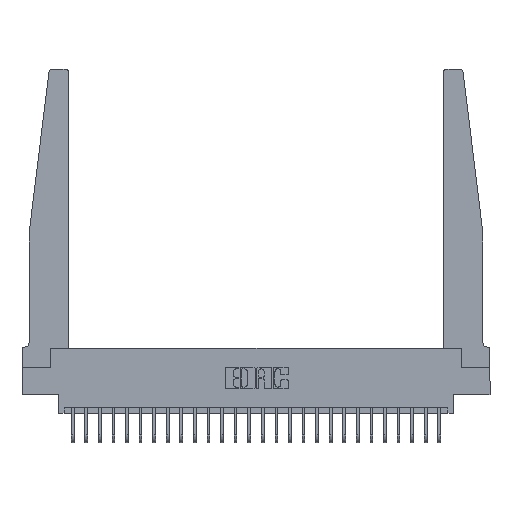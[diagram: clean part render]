
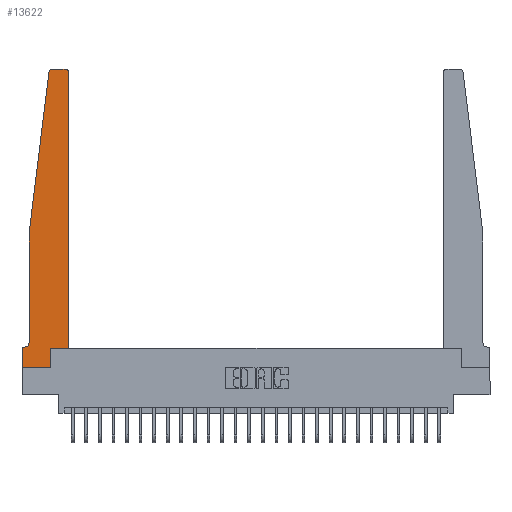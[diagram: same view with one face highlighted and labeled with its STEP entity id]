
A CAD part, top view. The second image highlights one B-rep face of the part: STEP entity #13622.
In plain terms, the highlighted planar face has unit normal (0, 0, 1).
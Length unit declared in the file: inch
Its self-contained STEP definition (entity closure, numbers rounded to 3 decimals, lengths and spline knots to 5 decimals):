
#13 = VERTEX_POINT ( 'NONE', #8820 ) ;
#181 = CIRCLE ( 'NONE', #4555, 0.03 ) ;
#565 = VERTEX_POINT ( 'NONE', #1072 ) ;
#1072 = CARTESIAN_POINT ( 'NONE',  ( 0.015, 0.1875, 0.37 ) ) ;
#1398 = DIRECTION ( 'NONE',  ( -1., 0., 0. ) ) ;
#1427 = EDGE_CURVE ( 'NONE', #3581, #565, #5714, .T. ) ;
#1668 = LINE ( 'NONE', #9292, #10512 ) ;
#1743 = VECTOR ( 'NONE', #21813, 39.37008 ) ;
#1884 = CARTESIAN_POINT ( 'NONE',  ( 0., 0.1875, 0.37 ) ) ;
#1920 = CARTESIAN_POINT ( 'NONE',  ( 0., 0.1875, 0.37 ) ) ;
#2096 = AXIS2_PLACEMENT_3D ( 'NONE', #1884, #16833, #5691 ) ;
#2272 = AXIS2_PLACEMENT_3D ( 'NONE', #2343, #15447, #4274 ) ;
#2343 = CARTESIAN_POINT ( 'NONE',  ( 0.395, 2.72, 0.37 ) ) ;
#2399 = EDGE_LOOP ( 'NONE', ( #18111, #4533, #22427, #10375, #23575, #20514, #14625, #22244, #3782, #5725, #24150, #6757 ) ) ;
#2478 = CARTESIAN_POINT ( 'NONE',  ( 0., 0., 0.37 ) ) ;
#2542 = VERTEX_POINT ( 'NONE', #15752 ) ;
#2615 = DIRECTION ( 'NONE',  ( 0., 1., 0. ) ) ;
#2855 = CARTESIAN_POINT ( 'NONE',  ( 0.2605, 0.18, 0.37 ) ) ;
#2891 = AXIS2_PLACEMENT_3D ( 'NONE', #23796, #12630, #1398 ) ;
#3581 = VERTEX_POINT ( 'NONE', #6512 ) ;
#3782 = ORIENTED_EDGE ( 'NONE', *, *, #17301, .T. ) ;
#4274 = DIRECTION ( 'NONE',  ( 1., 0., 0. ) ) ;
#4403 = LINE ( 'NONE', #24084, #13757 ) ;
#4533 = ORIENTED_EDGE ( 'NONE', *, *, #9156, .T. ) ;
#4555 = AXIS2_PLACEMENT_3D ( 'NONE', #21303, #10158, #23158 ) ;
#5691 = DIRECTION ( 'NONE',  ( 1., 0., 0. ) ) ;
#5714 = CIRCLE ( 'NONE', #2891, 0.05 ) ;
#5725 = ORIENTED_EDGE ( 'NONE', *, *, #6990, .T. ) ;
#6512 = CARTESIAN_POINT ( 'NONE',  ( 0.065, 0.2375, 0.37 ) ) ;
#6757 = ORIENTED_EDGE ( 'NONE', *, *, #15406, .T. ) ;
#6932 = CARTESIAN_POINT ( 'NONE',  ( 0.065, 1.25, 0.37 ) ) ;
#6990 = EDGE_CURVE ( 'NONE', #18319, #23135, #1668, .T. ) ;
#7347 = CIRCLE ( 'NONE', #2272, 0.03 ) ;
#7764 = DIRECTION ( 'NONE',  ( -1., 0., 0. ) ) ;
#7859 = EDGE_CURVE ( 'NONE', #23135, #17524, #22095, .T. ) ;
#8221 = EDGE_CURVE ( 'NONE', #20959, #3581, #23834, .T. ) ;
#8595 = CARTESIAN_POINT ( 'NONE',  ( 0.425, 0.18, 0.37 ) ) ;
#8820 = CARTESIAN_POINT ( 'NONE',  ( 0.27653, 2.75, 0.37 ) ) ;
#8822 = DIRECTION ( 'NONE',  ( -0.122, -0.992, 0. ) ) ;
#9156 = EDGE_CURVE ( 'NONE', #13, #15855, #181, .T. ) ;
#9198 = DIRECTION ( 'NONE',  ( -1., 0., 0. ) ) ;
#9292 = CARTESIAN_POINT ( 'NONE',  ( 0.425, 0.18, 0.37 ) ) ;
#10158 = DIRECTION ( 'NONE',  ( 0., 0., 1. ) ) ;
#10375 = ORIENTED_EDGE ( 'NONE', *, *, #8221, .T. ) ;
#10512 = VECTOR ( 'NONE', #11164, 39.37008 ) ;
#10900 = VERTEX_POINT ( 'NONE', #21131 ) ;
#11164 = DIRECTION ( 'NONE',  ( 1., 0., 0. ) ) ;
#11226 = CARTESIAN_POINT ( 'NONE',  ( 0.24675, 2.72367, 0.37 ) ) ;
#11274 = VERTEX_POINT ( 'NONE', #1920 ) ;
#11756 = VECTOR ( 'NONE', #8822, 39.37008 ) ;
#12276 = DIRECTION ( 'NONE',  ( 0., 1., 0. ) ) ;
#12317 = LINE ( 'NONE', #16188, #1743 ) ;
#12630 = DIRECTION ( 'NONE',  ( 0., 0., -1. ) ) ;
#12728 = EDGE_CURVE ( 'NONE', #11274, #10900, #14408, .T. ) ;
#13622 = ADVANCED_FACE ( 'NONE', ( #19303 ), #14972, .T. ) ;
#13757 = VECTOR ( 'NONE', #9198, 39.37008 ) ;
#13917 = VECTOR ( 'NONE', #18625, 39.37008 ) ;
#13948 = CARTESIAN_POINT ( 'NONE',  ( 0.065, 1.25, 0.37 ) ) ;
#14148 = EDGE_CURVE ( 'NONE', #565, #11274, #4403, .T. ) ;
#14408 = LINE ( 'NONE', #2478, #14991 ) ;
#14625 = ORIENTED_EDGE ( 'NONE', *, *, #12728, .T. ) ;
#14858 = CARTESIAN_POINT ( 'NONE',  ( 0.425, 2.72, 0.37 ) ) ;
#14972 = PLANE ( 'NONE',  #2096 ) ;
#14991 = VECTOR ( 'NONE', #20969, 39.37008 ) ;
#15242 = CARTESIAN_POINT ( 'NONE',  ( 0.2605, 0., 0.37 ) ) ;
#15353 = VECTOR ( 'NONE', #7764, 39.37008 ) ;
#15406 = EDGE_CURVE ( 'NONE', #17524, #2542, #7347, .T. ) ;
#15447 = DIRECTION ( 'NONE',  ( 0., 0., 1. ) ) ;
#15752 = CARTESIAN_POINT ( 'NONE',  ( 0.395, 2.75, 0.37 ) ) ;
#15855 = VERTEX_POINT ( 'NONE', #11226 ) ;
#16188 = CARTESIAN_POINT ( 'NONE',  ( 0., 0., 0.37 ) ) ;
#16766 = CARTESIAN_POINT ( 'NONE',  ( 0.065, 1.25, 0.37 ) ) ;
#16833 = DIRECTION ( 'NONE',  ( 0., 0., 1. ) ) ;
#17010 = CARTESIAN_POINT ( 'NONE',  ( 0.25, 2.75, 0.37 ) ) ;
#17301 = EDGE_CURVE ( 'NONE', #23055, #18319, #22741, .T. ) ;
#17489 = CARTESIAN_POINT ( 'NONE',  ( 0.425, 0.18, 0.37 ) ) ;
#17524 = VERTEX_POINT ( 'NONE', #14858 ) ;
#18111 = ORIENTED_EDGE ( 'NONE', *, *, #21391, .T. ) ;
#18319 = VERTEX_POINT ( 'NONE', #2855 ) ;
#18625 = DIRECTION ( 'NONE',  ( 0., -1., 0. ) ) ;
#19303 = FACE_OUTER_BOUND ( 'NONE', #2399, .T. ) ;
#19668 = CARTESIAN_POINT ( 'NONE',  ( 0.2605, 0.18, 0.37 ) ) ;
#20303 = LINE ( 'NONE', #17010, #15353 ) ;
#20514 = ORIENTED_EDGE ( 'NONE', *, *, #14148, .T. ) ;
#20959 = VERTEX_POINT ( 'NONE', #13948 ) ;
#20969 = DIRECTION ( 'NONE',  ( 0., -1., 0. ) ) ;
#21131 = CARTESIAN_POINT ( 'NONE',  ( 0., 0., 0.37 ) ) ;
#21303 = CARTESIAN_POINT ( 'NONE',  ( 0.27653, 2.72, 0.37 ) ) ;
#21391 = EDGE_CURVE ( 'NONE', #2542, #13, #20303, .T. ) ;
#21506 = VECTOR ( 'NONE', #2615, 39.37008 ) ;
#21619 = LINE ( 'NONE', #6932, #11756 ) ;
#21813 = DIRECTION ( 'NONE',  ( 1., 0., 0. ) ) ;
#22095 = LINE ( 'NONE', #17489, #21506 ) ;
#22244 = ORIENTED_EDGE ( 'NONE', *, *, #23899, .T. ) ;
#22427 = ORIENTED_EDGE ( 'NONE', *, *, #23893, .T. ) ;
#22741 = LINE ( 'NONE', #19668, #23313 ) ;
#23055 = VERTEX_POINT ( 'NONE', #15242 ) ;
#23135 = VERTEX_POINT ( 'NONE', #8595 ) ;
#23158 = DIRECTION ( 'NONE',  ( 1., 0., 0. ) ) ;
#23313 = VECTOR ( 'NONE', #12276, 39.37008 ) ;
#23575 = ORIENTED_EDGE ( 'NONE', *, *, #1427, .T. ) ;
#23796 = CARTESIAN_POINT ( 'NONE',  ( 0.015, 0.2375, 0.37 ) ) ;
#23834 = LINE ( 'NONE', #16766, #13917 ) ;
#23893 = EDGE_CURVE ( 'NONE', #15855, #20959, #21619, .T. ) ;
#23899 = EDGE_CURVE ( 'NONE', #10900, #23055, #12317, .T. ) ;
#24084 = CARTESIAN_POINT ( 'NONE',  ( 0.065, 0.1875, 0.37 ) ) ;
#24150 = ORIENTED_EDGE ( 'NONE', *, *, #7859, .T. ) ;
